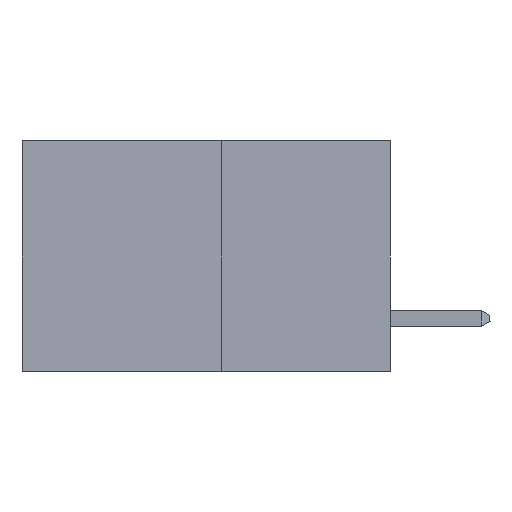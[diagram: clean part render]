
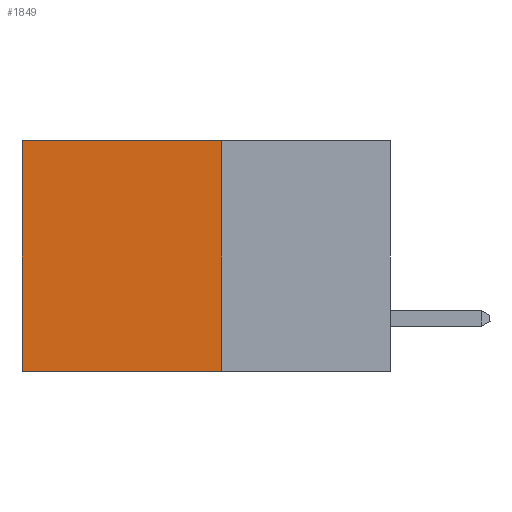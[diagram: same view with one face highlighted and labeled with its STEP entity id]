
A CAD part, left-side view. The second image highlights one B-rep face of the part: STEP entity #1849.
In plain terms, the highlighted planar face has unit normal (-1, 0, 0).
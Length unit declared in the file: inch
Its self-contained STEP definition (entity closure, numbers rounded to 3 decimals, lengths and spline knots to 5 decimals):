
#504 = CARTESIAN_POINT ( 'NONE',  ( 0.277, 0.59, -0.37 ) ) ;
#1026 = VERTEX_POINT ( 'NONE', #3461 ) ;
#1493 = DIRECTION ( 'NONE',  ( 0., 0., -1. ) ) ;
#1770 = EDGE_CURVE ( 'NONE', #9761, #11353, #10891, .T. ) ;
#1849 = ADVANCED_FACE ( 'NONE', ( #11871 ), #11302, .F. ) ;
#1894 = CARTESIAN_POINT ( 'NONE',  ( 0.277, 0.27, -0.37 ) ) ;
#3461 = CARTESIAN_POINT ( 'NONE',  ( 0.277, 0.27, 0. ) ) ;
#3751 = CARTESIAN_POINT ( 'NONE',  ( 0.277, 0.59, -0.37 ) ) ;
#3777 = EDGE_CURVE ( 'NONE', #10757, #11353, #9558, .T. ) ;
#3904 = DIRECTION ( 'NONE',  ( 0., 0., -1. ) ) ;
#4115 = DIRECTION ( 'NONE',  ( 0., 1., 0. ) ) ;
#4386 = CARTESIAN_POINT ( 'NONE',  ( 0.277, 0.27, -0.37 ) ) ;
#4551 = VECTOR ( 'NONE', #3904, 39.37008 ) ;
#4554 = EDGE_LOOP ( 'NONE', ( #7191, #10521, #9964, #5894 ) ) ;
#4945 = DIRECTION ( 'NONE',  ( 0., 1., 0. ) ) ;
#5056 = DIRECTION ( 'NONE',  ( 0., 0., -1. ) ) ;
#5159 = LINE ( 'NONE', #4386, #9573 ) ;
#5397 = CARTESIAN_POINT ( 'NONE',  ( 0.277, 0.59, 0. ) ) ;
#5520 = AXIS2_PLACEMENT_3D ( 'NONE', #1894, #6235, #5056 ) ;
#5894 = ORIENTED_EDGE ( 'NONE', *, *, #11058, .T. ) ;
#6189 = LINE ( 'NONE', #10537, #11114 ) ;
#6235 = DIRECTION ( 'NONE',  ( 1., 0., 0. ) ) ;
#6601 = CARTESIAN_POINT ( 'NONE',  ( 0.277, 0.27, -0.37 ) ) ;
#7191 = ORIENTED_EDGE ( 'NONE', *, *, #3777, .T. ) ;
#9195 = CARTESIAN_POINT ( 'NONE',  ( 0.277, 0.27, -0.37 ) ) ;
#9528 = EDGE_CURVE ( 'NONE', #1026, #9761, #5159, .T. ) ;
#9558 = LINE ( 'NONE', #3751, #4551 ) ;
#9573 = VECTOR ( 'NONE', #1493, 39.37008 ) ;
#9761 = VERTEX_POINT ( 'NONE', #6601 ) ;
#9964 = ORIENTED_EDGE ( 'NONE', *, *, #9528, .F. ) ;
#10521 = ORIENTED_EDGE ( 'NONE', *, *, #1770, .F. ) ;
#10537 = CARTESIAN_POINT ( 'NONE',  ( 0.277, 0.27, 0. ) ) ;
#10614 = VECTOR ( 'NONE', #4115, 39.37008 ) ;
#10757 = VERTEX_POINT ( 'NONE', #5397 ) ;
#10891 = LINE ( 'NONE', #9195, #10614 ) ;
#11058 = EDGE_CURVE ( 'NONE', #1026, #10757, #6189, .T. ) ;
#11114 = VECTOR ( 'NONE', #4945, 39.37008 ) ;
#11302 = PLANE ( 'NONE',  #5520 ) ;
#11353 = VERTEX_POINT ( 'NONE', #504 ) ;
#11871 = FACE_OUTER_BOUND ( 'NONE', #4554, .T. ) ;
